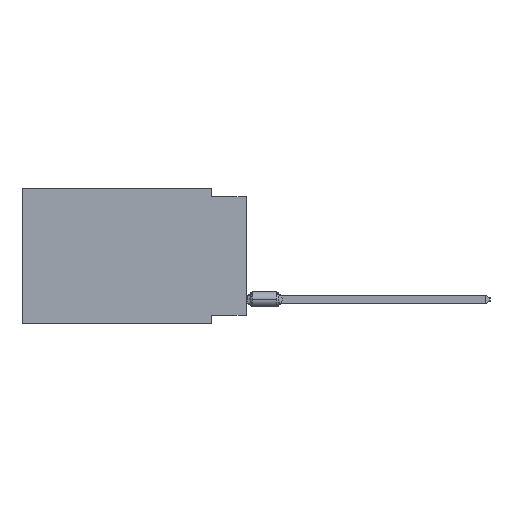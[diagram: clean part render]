
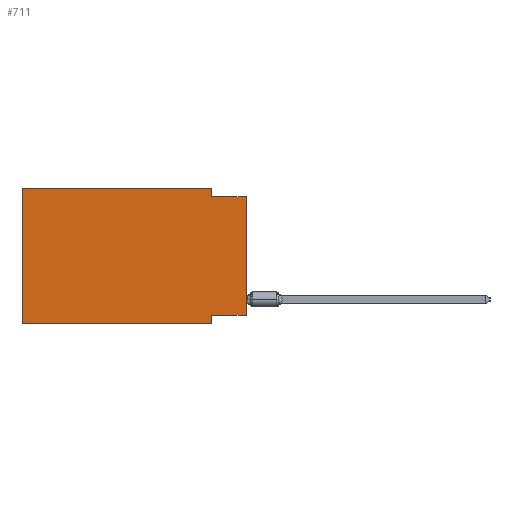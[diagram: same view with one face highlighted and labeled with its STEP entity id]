
A CAD part, left-side view. The second image highlights one B-rep face of the part: STEP entity #711.
In plain terms, the highlighted planar face has unit normal (-1, 0, 0).
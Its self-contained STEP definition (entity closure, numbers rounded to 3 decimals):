
#3 = VERTEX_POINT ( 'NONE', #15678 ) ;
#78 = LINE ( 'NONE', #31722, #12437 ) ;
#258 = ORIENTED_EDGE ( 'NONE', *, *, #38556, .F. ) ;
#484 = ORIENTED_EDGE ( 'NONE', *, *, #14280, .T. ) ;
#711 = ADVANCED_FACE ( 'NONE', ( #18970 ), #18682, .F. ) ;
#942 = DIRECTION ( 'NONE',  ( 0., 0., -1. ) ) ;
#1096 = DIRECTION ( 'NONE',  ( 0., 0., -1. ) ) ;
#4055 = ORIENTED_EDGE ( 'NONE', *, *, #9255, .F. ) ;
#4329 = AXIS2_PLACEMENT_3D ( 'NONE', #36558, #46228, #54463 ) ;
#5693 = LINE ( 'NONE', #41158, #39518 ) ;
#6760 = DIRECTION ( 'NONE',  ( 0., 0., 1. ) ) ;
#6993 = EDGE_CURVE ( 'NONE', #42844, #3, #42525, .T. ) ;
#8269 = EDGE_CURVE ( 'NONE', #14168, #57120, #78, .T. ) ;
#9255 = EDGE_CURVE ( 'NONE', #3, #48783, #55621, .T. ) ;
#10261 = ORIENTED_EDGE ( 'NONE', *, *, #11162, .F. ) ;
#10649 = EDGE_CURVE ( 'NONE', #42844, #22022, #50166, .T. ) ;
#11162 = EDGE_CURVE ( 'NONE', #11849, #13084, #34799, .T. ) ;
#11618 = CARTESIAN_POINT ( 'NONE',  ( 0., 16.383, -9.906 ) ) ;
#11849 = VERTEX_POINT ( 'NONE', #11618 ) ;
#12437 = VECTOR ( 'NONE', #942, 1000. ) ;
#13084 = VERTEX_POINT ( 'NONE', #57076 ) ;
#13106 = CARTESIAN_POINT ( 'NONE',  ( 0., 16.383, 0. ) ) ;
#14168 = VERTEX_POINT ( 'NONE', #19673 ) ;
#14280 = EDGE_CURVE ( 'NONE', #11849, #48783, #20525, .T. ) ;
#15678 = CARTESIAN_POINT ( 'NONE',  ( 0., 2.54, -9.271 ) ) ;
#18682 = PLANE ( 'NONE',  #4329 ) ;
#18816 = CARTESIAN_POINT ( 'NONE',  ( 0., 0., -0.635 ) ) ;
#18970 = FACE_OUTER_BOUND ( 'NONE', #31642, .T. ) ;
#19100 = LINE ( 'NONE', #36973, #52556 ) ;
#19159 = ORIENTED_EDGE ( 'NONE', *, *, #6993, .F. ) ;
#19455 = DIRECTION ( 'NONE',  ( 0., -1., 0. ) ) ;
#19673 = CARTESIAN_POINT ( 'NONE',  ( 0., 2.54, 0. ) ) ;
#20525 = LINE ( 'NONE', #24655, #48585 ) ;
#22022 = VERTEX_POINT ( 'NONE', #18816 ) ;
#23801 = DIRECTION ( 'NONE',  ( 0., -1., 0. ) ) ;
#24655 = CARTESIAN_POINT ( 'NONE',  ( 0., 16.383, -9.906 ) ) ;
#25805 = DIRECTION ( 'NONE',  ( 0., 1., 0. ) ) ;
#29740 = ORIENTED_EDGE ( 'NONE', *, *, #56130, .F. ) ;
#31642 = EDGE_LOOP ( 'NONE', ( #56795, #258, #34241, #29740, #10261, #484, #4055, #19159 ) ) ;
#31722 = CARTESIAN_POINT ( 'NONE',  ( 0., 2.54, 0. ) ) ;
#32201 = CARTESIAN_POINT ( 'NONE',  ( 0., 0., -9.271 ) ) ;
#33437 = DIRECTION ( 'NONE',  ( 0., -1., 0. ) ) ;
#34241 = ORIENTED_EDGE ( 'NONE', *, *, #8269, .F. ) ;
#34799 = LINE ( 'NONE', #13106, #36872 ) ;
#36558 = CARTESIAN_POINT ( 'NONE',  ( 0., 16.383, 0. ) ) ;
#36872 = VECTOR ( 'NONE', #49967, 1000. ) ;
#36973 = CARTESIAN_POINT ( 'NONE',  ( 0., 0., -0.635 ) ) ;
#37490 = VECTOR ( 'NONE', #25805, 1000. ) ;
#38556 = EDGE_CURVE ( 'NONE', #57120, #22022, #19100, .T. ) ;
#39502 = CARTESIAN_POINT ( 'NONE',  ( 0., 2.54, -0.635 ) ) ;
#39518 = VECTOR ( 'NONE', #19455, 1000. ) ;
#41158 = CARTESIAN_POINT ( 'NONE',  ( 0., 16.383, 0. ) ) ;
#42525 = LINE ( 'NONE', #52779, #37490 ) ;
#42844 = VERTEX_POINT ( 'NONE', #32201 ) ;
#45240 = VECTOR ( 'NONE', #1096, 1000. ) ;
#46228 = DIRECTION ( 'NONE',  ( 1., 0., 0. ) ) ;
#46229 = CARTESIAN_POINT ( 'NONE',  ( 0., 2.54, -9.906 ) ) ;
#46910 = CARTESIAN_POINT ( 'NONE',  ( 0., 0., 0. ) ) ;
#48585 = VECTOR ( 'NONE', #33437, 1000. ) ;
#48783 = VERTEX_POINT ( 'NONE', #52740 ) ;
#49967 = DIRECTION ( 'NONE',  ( 0., 0., 1. ) ) ;
#50166 = LINE ( 'NONE', #46910, #50862 ) ;
#50862 = VECTOR ( 'NONE', #6760, 1000. ) ;
#52556 = VECTOR ( 'NONE', #23801, 1000. ) ;
#52740 = CARTESIAN_POINT ( 'NONE',  ( 0., 2.54, -9.906 ) ) ;
#52779 = CARTESIAN_POINT ( 'NONE',  ( 0., 0., -9.271 ) ) ;
#54463 = DIRECTION ( 'NONE',  ( 0., 0., -1. ) ) ;
#55621 = LINE ( 'NONE', #46229, #45240 ) ;
#56130 = EDGE_CURVE ( 'NONE', #13084, #14168, #5693, .T. ) ;
#56795 = ORIENTED_EDGE ( 'NONE', *, *, #10649, .T. ) ;
#57076 = CARTESIAN_POINT ( 'NONE',  ( 0., 16.383, 0. ) ) ;
#57120 = VERTEX_POINT ( 'NONE', #39502 ) ;
